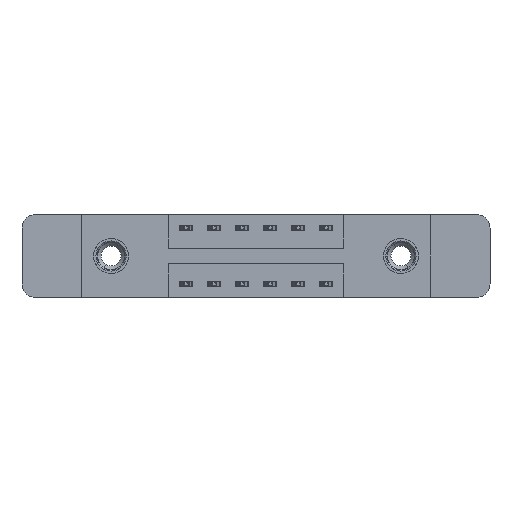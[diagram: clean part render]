
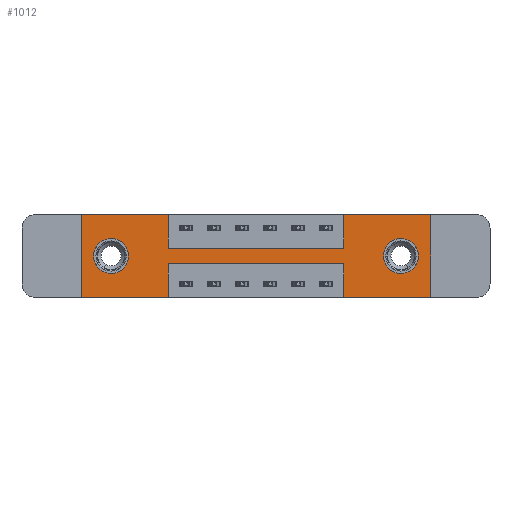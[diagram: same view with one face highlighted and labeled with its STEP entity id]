
A CAD part, front view. The second image highlights one B-rep face of the part: STEP entity #1012.
In plain terms, the highlighted planar face has unit normal (0, -1, 0).
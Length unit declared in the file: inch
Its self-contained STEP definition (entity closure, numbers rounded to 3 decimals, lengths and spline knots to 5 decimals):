
#343 = ORIENTED_EDGE ( 'NONE', *, *, #7823, .F. ) ;
#349 = VERTEX_POINT ( 'NONE', #12912 ) ;
#470 = ORIENTED_EDGE ( 'NONE', *, *, #12723, .F. ) ;
#600 = CARTESIAN_POINT ( 'NONE',  ( 1.1725, 0., 0. ) ) ;
#662 = DIRECTION ( 'NONE',  ( -1., 0., 0. ) ) ;
#959 = DIRECTION ( 'NONE',  ( 0., 0., -1. ) ) ;
#1012 = ADVANCED_FACE ( 'NONE', ( #9797, #5154, #9456 ), #9513, .T. ) ;
#1136 = CARTESIAN_POINT ( 'NONE',  ( 0.3875, 0., 0. ) ) ;
#1384 = ORIENTED_EDGE ( 'NONE', *, *, #7632, .F. ) ;
#1591 = EDGE_CURVE ( 'NONE', #2443, #4121, #11591, .T. ) ;
#1646 = VECTOR ( 'NONE', #8244, 39.37008 ) ;
#1750 = DIRECTION ( 'NONE',  ( -1., 0., 0. ) ) ;
#1835 = CARTESIAN_POINT ( 'NONE',  ( 1.56, 0., -0.37 ) ) ;
#1870 = CIRCLE ( 'NONE', #5673, 0.078 ) ;
#1998 = VERTEX_POINT ( 'NONE', #7686 ) ;
#2198 = CARTESIAN_POINT ( 'NONE',  ( 1.56, 0., 0. ) ) ;
#2218 = ORIENTED_EDGE ( 'NONE', *, *, #1591, .F. ) ;
#2360 = EDGE_LOOP ( 'NONE', ( #9590, #9662 ) ) ;
#2436 = VECTOR ( 'NONE', #8452, 39.37008 ) ;
#2443 = VERTEX_POINT ( 'NONE', #1136 ) ;
#2444 = EDGE_CURVE ( 'NONE', #6264, #7062, #8070, .T. ) ;
#2663 = CARTESIAN_POINT ( 'NONE',  ( 0., 0., 0. ) ) ;
#2756 = EDGE_CURVE ( 'NONE', #3851, #4421, #1870, .T. ) ;
#2785 = DIRECTION ( 'NONE',  ( 0., -1., 0. ) ) ;
#2964 = CARTESIAN_POINT ( 'NONE',  ( 0., 0., -0.37 ) ) ;
#3046 = VERTEX_POINT ( 'NONE', #11462 ) ;
#3141 = DIRECTION ( 'NONE',  ( 1., 0., 0. ) ) ;
#3176 = VERTEX_POINT ( 'NONE', #5521 ) ;
#3393 = ORIENTED_EDGE ( 'NONE', *, *, #7808, .F. ) ;
#3395 = CARTESIAN_POINT ( 'NONE',  ( 1.4275, 0., -0.185 ) ) ;
#3462 = CARTESIAN_POINT ( 'NONE',  ( 0.3875, 0., 0. ) ) ;
#3494 = CIRCLE ( 'NONE', #9089, 0.078 ) ;
#3755 = LINE ( 'NONE', #600, #8885 ) ;
#3851 = VERTEX_POINT ( 'NONE', #9527 ) ;
#4118 = CARTESIAN_POINT ( 'NONE',  ( 1.4275, 0., -0.185 ) ) ;
#4121 = VERTEX_POINT ( 'NONE', #4862 ) ;
#4242 = DIRECTION ( 'NONE',  ( 0., 0., -1. ) ) ;
#4289 = VECTOR ( 'NONE', #662, 39.37008 ) ;
#4421 = VERTEX_POINT ( 'NONE', #10879 ) ;
#4433 = CARTESIAN_POINT ( 'NONE',  ( 1.4275, 0., -0.107 ) ) ;
#4834 = DIRECTION ( 'NONE',  ( -1., 0., 0. ) ) ;
#4862 = CARTESIAN_POINT ( 'NONE',  ( 0.3875, 0., -0.15 ) ) ;
#4940 = EDGE_CURVE ( 'NONE', #7604, #6264, #9318, .T. ) ;
#5046 = EDGE_CURVE ( 'NONE', #3046, #13980, #3494, .T. ) ;
#5116 = VECTOR ( 'NONE', #959, 39.37008 ) ;
#5154 = FACE_BOUND ( 'NONE', #2360, .T. ) ;
#5163 = CIRCLE ( 'NONE', #6910, 0.078 ) ;
#5203 = DIRECTION ( 'NONE',  ( 0., 1., 0. ) ) ;
#5521 = CARTESIAN_POINT ( 'NONE',  ( 0.3875, 0., -0.22 ) ) ;
#5534 = EDGE_CURVE ( 'NONE', #3176, #9566, #7581, .T. ) ;
#5611 = ORIENTED_EDGE ( 'NONE', *, *, #7046, .T. ) ;
#5648 = VERTEX_POINT ( 'NONE', #13926 ) ;
#5669 = DIRECTION ( 'NONE',  ( 0., 1., 0. ) ) ;
#5673 = AXIS2_PLACEMENT_3D ( 'NONE', #10351, #7535, #10806 ) ;
#6264 = VERTEX_POINT ( 'NONE', #9959 ) ;
#6392 = CARTESIAN_POINT ( 'NONE',  ( 1.1725, 0., -0.37 ) ) ;
#6450 = EDGE_CURVE ( 'NONE', #9566, #5648, #9685, .T. ) ;
#6522 = LINE ( 'NONE', #7305, #6706 ) ;
#6699 = CIRCLE ( 'NONE', #8757, 0.078 ) ;
#6706 = VECTOR ( 'NONE', #13593, 39.37008 ) ;
#6784 = VECTOR ( 'NONE', #1750, 39.37008 ) ;
#6805 = ORIENTED_EDGE ( 'NONE', *, *, #11142, .F. ) ;
#6910 = AXIS2_PLACEMENT_3D ( 'NONE', #8418, #5203, #10744 ) ;
#6934 = ORIENTED_EDGE ( 'NONE', *, *, #6450, .F. ) ;
#7046 = EDGE_CURVE ( 'NONE', #13980, #3046, #6699, .T. ) ;
#7062 = VERTEX_POINT ( 'NONE', #1835 ) ;
#7172 = ORIENTED_EDGE ( 'NONE', *, *, #2444, .F. ) ;
#7242 = CARTESIAN_POINT ( 'NONE',  ( 0., 0., -0.37 ) ) ;
#7305 = CARTESIAN_POINT ( 'NONE',  ( 0., 0., 0. ) ) ;
#7535 = DIRECTION ( 'NONE',  ( 0., 1., 0. ) ) ;
#7581 = LINE ( 'NONE', #12555, #9792 ) ;
#7604 = VERTEX_POINT ( 'NONE', #11796 ) ;
#7632 = EDGE_CURVE ( 'NONE', #349, #1998, #12946, .T. ) ;
#7686 = CARTESIAN_POINT ( 'NONE',  ( 1.1725, 0., -0.22 ) ) ;
#7808 = EDGE_CURVE ( 'NONE', #1998, #3176, #11927, .T. ) ;
#7823 = EDGE_CURVE ( 'NONE', #5648, #8558, #6522, .T. ) ;
#7878 = CARTESIAN_POINT ( 'NONE',  ( 1.1725, 0., -0.15 ) ) ;
#7918 = VECTOR ( 'NONE', #13441, 39.37008 ) ;
#8070 = LINE ( 'NONE', #2198, #5116 ) ;
#8244 = DIRECTION ( 'NONE',  ( 1., 0., 0. ) ) ;
#8418 = CARTESIAN_POINT ( 'NONE',  ( 0.1325, 0., -0.185 ) ) ;
#8441 = CARTESIAN_POINT ( 'NONE',  ( 0.3875, 0., -0.22 ) ) ;
#8452 = DIRECTION ( 'NONE',  ( 0., 0., 1. ) ) ;
#8558 = VERTEX_POINT ( 'NONE', #12357 ) ;
#8757 = AXIS2_PLACEMENT_3D ( 'NONE', #4118, #9523, #9663 ) ;
#8885 = VECTOR ( 'NONE', #10201, 39.37008 ) ;
#9025 = VERTEX_POINT ( 'NONE', #7878 ) ;
#9046 = DIRECTION ( 'NONE',  ( 0., 0., -1. ) ) ;
#9089 = AXIS2_PLACEMENT_3D ( 'NONE', #3395, #5669, #4242 ) ;
#9318 = LINE ( 'NONE', #2663, #1646 ) ;
#9456 = FACE_OUTER_BOUND ( 'NONE', #11233, .T. ) ;
#9513 = PLANE ( 'NONE',  #12123 ) ;
#9523 = DIRECTION ( 'NONE',  ( 0., 1., 0. ) ) ;
#9527 = CARTESIAN_POINT ( 'NONE',  ( 0.1325, 0., -0.263 ) ) ;
#9566 = VERTEX_POINT ( 'NONE', #12037 ) ;
#9590 = ORIENTED_EDGE ( 'NONE', *, *, #10408, .T. ) ;
#9662 = ORIENTED_EDGE ( 'NONE', *, *, #2756, .T. ) ;
#9663 = DIRECTION ( 'NONE',  ( 0., 0., -1. ) ) ;
#9685 = LINE ( 'NONE', #7242, #6784 ) ;
#9713 = EDGE_CURVE ( 'NONE', #4121, #9025, #12313, .T. ) ;
#9792 = VECTOR ( 'NONE', #10829, 39.37008 ) ;
#9797 = FACE_BOUND ( 'NONE', #13599, .T. ) ;
#9915 = ORIENTED_EDGE ( 'NONE', *, *, #10062, .F. ) ;
#9959 = CARTESIAN_POINT ( 'NONE',  ( 1.56, 0., 0. ) ) ;
#10062 = EDGE_CURVE ( 'NONE', #7062, #349, #11042, .T. ) ;
#10201 = DIRECTION ( 'NONE',  ( 0., 0., 1. ) ) ;
#10351 = CARTESIAN_POINT ( 'NONE',  ( 0.1325, 0., -0.185 ) ) ;
#10408 = EDGE_CURVE ( 'NONE', #4421, #3851, #5163, .T. ) ;
#10744 = DIRECTION ( 'NONE',  ( 0., 0., 1. ) ) ;
#10794 = LINE ( 'NONE', #13981, #12956 ) ;
#10806 = DIRECTION ( 'NONE',  ( 0., 0., 1. ) ) ;
#10829 = DIRECTION ( 'NONE',  ( 0., 0., -1. ) ) ;
#10879 = CARTESIAN_POINT ( 'NONE',  ( 0.1325, 0., -0.107 ) ) ;
#10881 = ORIENTED_EDGE ( 'NONE', *, *, #5046, .T. ) ;
#11042 = LINE ( 'NONE', #12393, #12523 ) ;
#11142 = EDGE_CURVE ( 'NONE', #9025, #7604, #3755, .T. ) ;
#11233 = EDGE_LOOP ( 'NONE', ( #13511, #3393, #1384, #9915, #7172, #13145, #6805, #13865, #2218, #470, #343, #6934 ) ) ;
#11462 = CARTESIAN_POINT ( 'NONE',  ( 1.4275, 0., -0.263 ) ) ;
#11591 = LINE ( 'NONE', #3462, #7918 ) ;
#11631 = DIRECTION ( 'NONE',  ( 1., 0., 0. ) ) ;
#11787 = CARTESIAN_POINT ( 'NONE',  ( 0.3875, 0., -0.15 ) ) ;
#11796 = CARTESIAN_POINT ( 'NONE',  ( 1.1725, 0., 0. ) ) ;
#11927 = LINE ( 'NONE', #8441, #4289 ) ;
#11965 = VECTOR ( 'NONE', #11631, 39.37008 ) ;
#12037 = CARTESIAN_POINT ( 'NONE',  ( 0.3875, 0., -0.37 ) ) ;
#12123 = AXIS2_PLACEMENT_3D ( 'NONE', #2964, #2785, #9046 ) ;
#12313 = LINE ( 'NONE', #11787, #11965 ) ;
#12357 = CARTESIAN_POINT ( 'NONE',  ( 0., 0., 0. ) ) ;
#12393 = CARTESIAN_POINT ( 'NONE',  ( 0., 0., -0.37 ) ) ;
#12523 = VECTOR ( 'NONE', #4834, 39.37008 ) ;
#12555 = CARTESIAN_POINT ( 'NONE',  ( 0.3875, 0., -0.37 ) ) ;
#12723 = EDGE_CURVE ( 'NONE', #8558, #2443, #10794, .T. ) ;
#12912 = CARTESIAN_POINT ( 'NONE',  ( 1.1725, 0., -0.37 ) ) ;
#12946 = LINE ( 'NONE', #6392, #2436 ) ;
#12956 = VECTOR ( 'NONE', #3141, 39.37008 ) ;
#13145 = ORIENTED_EDGE ( 'NONE', *, *, #4940, .F. ) ;
#13441 = DIRECTION ( 'NONE',  ( 0., 0., -1. ) ) ;
#13511 = ORIENTED_EDGE ( 'NONE', *, *, #5534, .F. ) ;
#13593 = DIRECTION ( 'NONE',  ( 0., 0., 1. ) ) ;
#13599 = EDGE_LOOP ( 'NONE', ( #5611, #10881 ) ) ;
#13865 = ORIENTED_EDGE ( 'NONE', *, *, #9713, .F. ) ;
#13926 = CARTESIAN_POINT ( 'NONE',  ( 0., 0., -0.37 ) ) ;
#13980 = VERTEX_POINT ( 'NONE', #4433 ) ;
#13981 = CARTESIAN_POINT ( 'NONE',  ( 0., 0., 0. ) ) ;
